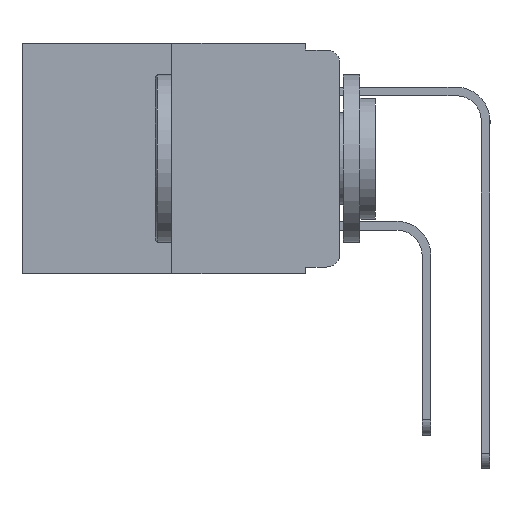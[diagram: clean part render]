
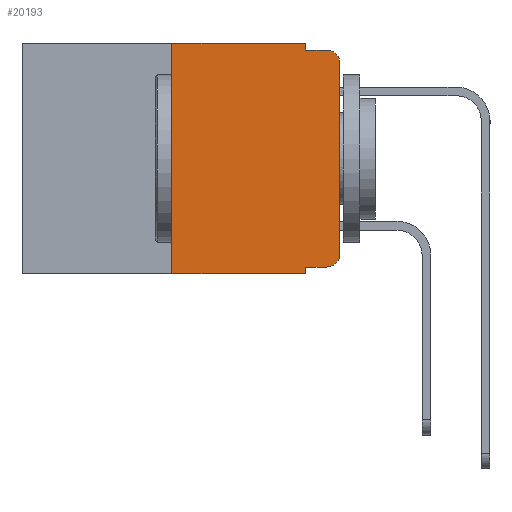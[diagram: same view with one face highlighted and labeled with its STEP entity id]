
A CAD part, left-side view. The second image highlights one B-rep face of the part: STEP entity #20193.
In plain terms, the highlighted planar face has unit normal (-1, 0, 0).
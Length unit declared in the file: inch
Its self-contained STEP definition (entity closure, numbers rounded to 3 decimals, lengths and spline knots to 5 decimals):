
#456 = LINE ( 'NONE', #9742, #17325 ) ;
#466 = AXIS2_PLACEMENT_3D ( 'NONE', #11135, #1274, #12730 ) ;
#998 = VERTEX_POINT ( 'NONE', #15380 ) ;
#1039 = CIRCLE ( 'NONE', #20882, 0.02 ) ;
#1091 = DIRECTION ( 'NONE',  ( 0., 0., 1. ) ) ;
#1274 = DIRECTION ( 'NONE',  ( -1., 0., 0. ) ) ;
#1431 = CARTESIAN_POINT ( 'NONE',  ( 0., 0.473, 0. ) ) ;
#1980 = VERTEX_POINT ( 'NONE', #15753 ) ;
#2075 = EDGE_CURVE ( 'NONE', #14745, #5424, #7371, .T. ) ;
#2133 = CARTESIAN_POINT ( 'NONE',  ( 0., 0., -0.313 ) ) ;
#2342 = CARTESIAN_POINT ( 'NONE',  ( 0., 0.051, 0. ) ) ;
#2518 = LINE ( 'NONE', #8297, #15489 ) ;
#2686 = DIRECTION ( 'NONE',  ( 0., 0., -1. ) ) ;
#3167 = VERTEX_POINT ( 'NONE', #2342 ) ;
#3268 = ORIENTED_EDGE ( 'NONE', *, *, #9382, .T. ) ;
#3995 = ORIENTED_EDGE ( 'NONE', *, *, #4966, .T. ) ;
#4326 = ORIENTED_EDGE ( 'NONE', *, *, #4682, .T. ) ;
#4682 = EDGE_CURVE ( 'NONE', #21070, #7852, #1039, .T. ) ;
#4810 = ORIENTED_EDGE ( 'NONE', *, *, #11947, .F. ) ;
#4951 = ORIENTED_EDGE ( 'NONE', *, *, #6901, .T. ) ;
#4966 = EDGE_CURVE ( 'NONE', #19309, #7816, #8030, .T. ) ;
#5271 = CARTESIAN_POINT ( 'NONE',  ( 0., 0., -0.03 ) ) ;
#5424 = VERTEX_POINT ( 'NONE', #15454 ) ;
#5949 = VECTOR ( 'NONE', #2686, 39.37008 ) ;
#6366 = LINE ( 'NONE', #20900, #13988 ) ;
#6461 = CARTESIAN_POINT ( 'NONE',  ( 0., 0.25, 0. ) ) ;
#6721 = DIRECTION ( 'NONE',  ( 0., 0., -1. ) ) ;
#6852 = ORIENTED_EDGE ( 'NONE', *, *, #10202, .F. ) ;
#6901 = EDGE_CURVE ( 'NONE', #1980, #21070, #6366, .T. ) ;
#7342 = ORIENTED_EDGE ( 'NONE', *, *, #9537, .T. ) ;
#7371 = LINE ( 'NONE', #6461, #15459 ) ;
#7474 = ORIENTED_EDGE ( 'NONE', *, *, #2075, .F. ) ;
#7720 = LINE ( 'NONE', #1431, #12025 ) ;
#7816 = VERTEX_POINT ( 'NONE', #11858 ) ;
#7852 = VERTEX_POINT ( 'NONE', #2133 ) ;
#7856 = PLANE ( 'NONE',  #16955 ) ;
#8030 = CIRCLE ( 'NONE', #466, 0.02 ) ;
#8297 = CARTESIAN_POINT ( 'NONE',  ( 0., 0.051, -0.01 ) ) ;
#8447 = VERTEX_POINT ( 'NONE', #18285 ) ;
#8454 = ORIENTED_EDGE ( 'NONE', *, *, #8709, .F. ) ;
#8500 = DIRECTION ( 'NONE',  ( 0., 0., -1. ) ) ;
#8517 = ORIENTED_EDGE ( 'NONE', *, *, #10039, .F. ) ;
#8543 = CARTESIAN_POINT ( 'NONE',  ( 0., 0.02, -0.333 ) ) ;
#8604 = CARTESIAN_POINT ( 'NONE',  ( 0., 0.02, -0.313 ) ) ;
#8709 = EDGE_CURVE ( 'NONE', #3167, #998, #17358, .T. ) ;
#8994 = VECTOR ( 'NONE', #6721, 39.37008 ) ;
#9326 = CARTESIAN_POINT ( 'NONE',  ( 0., 0., 0. ) ) ;
#9382 = EDGE_CURVE ( 'NONE', #7852, #19309, #12305, .T. ) ;
#9457 = EDGE_LOOP ( 'NONE', ( #3268, #3995, #4810, #8454, #8517, #7474, #7342, #6852, #4951, #4326 ) ) ;
#9491 = DIRECTION ( 'NONE',  ( 1., 0., 0. ) ) ;
#9537 = EDGE_CURVE ( 'NONE', #14745, #8447, #456, .T. ) ;
#9742 = CARTESIAN_POINT ( 'NONE',  ( 0., 0.473, -0.343 ) ) ;
#10039 = EDGE_CURVE ( 'NONE', #5424, #3167, #7720, .T. ) ;
#10202 = EDGE_CURVE ( 'NONE', #1980, #8447, #13760, .T. ) ;
#11135 = CARTESIAN_POINT ( 'NONE',  ( 0., 0.02, -0.03 ) ) ;
#11858 = CARTESIAN_POINT ( 'NONE',  ( 0., 0.02, -0.01 ) ) ;
#11947 = EDGE_CURVE ( 'NONE', #998, #7816, #2518, .T. ) ;
#12025 = VECTOR ( 'NONE', #12885, 39.37008 ) ;
#12305 = LINE ( 'NONE', #9326, #20328 ) ;
#12730 = DIRECTION ( 'NONE',  ( 0., 0., -1. ) ) ;
#12885 = DIRECTION ( 'NONE',  ( 0., -1., 0. ) ) ;
#12939 = DIRECTION ( 'NONE',  ( 0., -1., 0. ) ) ;
#13760 = LINE ( 'NONE', #18088, #8994 ) ;
#13988 = VECTOR ( 'NONE', #12939, 39.37008 ) ;
#14065 = CARTESIAN_POINT ( 'NONE',  ( 0., 0.051, 0. ) ) ;
#14629 = DIRECTION ( 'NONE',  ( -1., 0., 0. ) ) ;
#14745 = VERTEX_POINT ( 'NONE', #15440 ) ;
#15380 = CARTESIAN_POINT ( 'NONE',  ( 0., 0.051, -0.01 ) ) ;
#15440 = CARTESIAN_POINT ( 'NONE',  ( 0., 0.25, -0.343 ) ) ;
#15454 = CARTESIAN_POINT ( 'NONE',  ( 0., 0.25, 0. ) ) ;
#15459 = VECTOR ( 'NONE', #20951, 39.37008 ) ;
#15489 = VECTOR ( 'NONE', #17928, 39.37008 ) ;
#15753 = CARTESIAN_POINT ( 'NONE',  ( 0., 0.051, -0.333 ) ) ;
#16218 = DIRECTION ( 'NONE',  ( 0., -1., 0. ) ) ;
#16955 = AXIS2_PLACEMENT_3D ( 'NONE', #19101, #9491, #20698 ) ;
#17325 = VECTOR ( 'NONE', #16218, 39.37008 ) ;
#17358 = LINE ( 'NONE', #14065, #5949 ) ;
#17928 = DIRECTION ( 'NONE',  ( 0., -1., 0. ) ) ;
#18088 = CARTESIAN_POINT ( 'NONE',  ( 0., 0.051, 0. ) ) ;
#18285 = CARTESIAN_POINT ( 'NONE',  ( 0., 0.051, -0.343 ) ) ;
#19101 = CARTESIAN_POINT ( 'NONE',  ( 0., 0.473, 0. ) ) ;
#19309 = VERTEX_POINT ( 'NONE', #5271 ) ;
#20193 = ADVANCED_FACE ( 'NONE', ( #20740 ), #7856, .F. ) ;
#20328 = VECTOR ( 'NONE', #1091, 39.37008 ) ;
#20698 = DIRECTION ( 'NONE',  ( 0., 0., -1. ) ) ;
#20740 = FACE_OUTER_BOUND ( 'NONE', #9457, .T. ) ;
#20882 = AXIS2_PLACEMENT_3D ( 'NONE', #8604, #14629, #8500 ) ;
#20900 = CARTESIAN_POINT ( 'NONE',  ( 0., 0.051, -0.333 ) ) ;
#20951 = DIRECTION ( 'NONE',  ( 0., 0., 1. ) ) ;
#21070 = VERTEX_POINT ( 'NONE', #8543 ) ;
